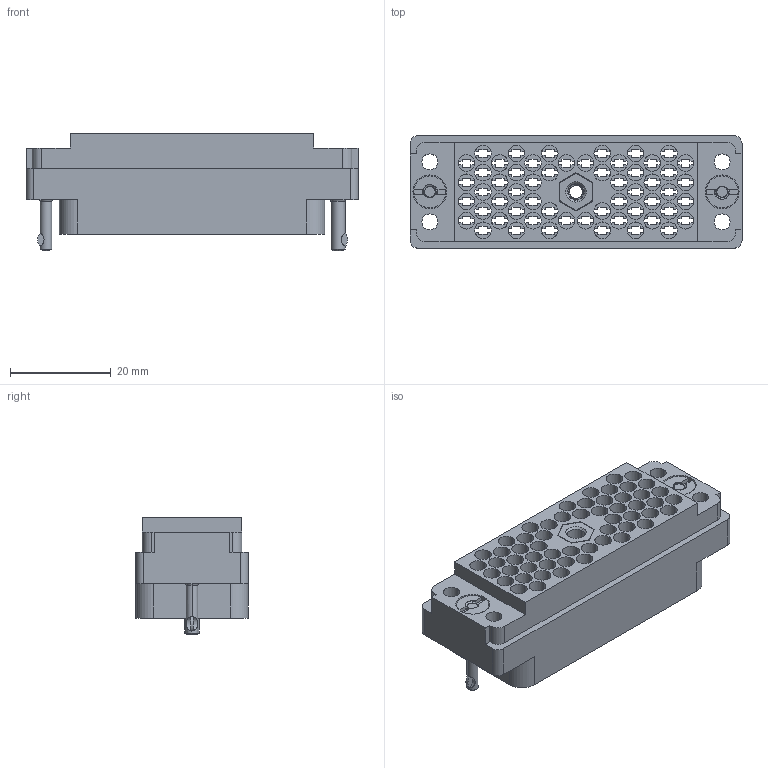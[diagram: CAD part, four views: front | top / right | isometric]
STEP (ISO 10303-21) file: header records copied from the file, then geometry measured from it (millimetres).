
FILE_DESCRIPTION (( 'STEP AP203' ), '1' );
FILE_NAME ('516-056-000-502.STEP', '2020-03-10T04:58:30', ( '' ), ( '' ), 'SwSTEP 2.0', 'SolidWorks 2016', '' );
FILE_SCHEMA (( 'CONFIG_CONTROL_DESIGN' ));
Length unit declared in the file: inch
Products named in the file (6): 516-222-038-102_057; 516-252-035-100_516-252-035-100; 516-252-021-102_056; 516-222-038-102_056; 516 Plug Insulator_056; 516-056-000-502
Assembly tree (6 placements, depth 2):
  516-056-000-502
    516 Plug Insulator_056
    516-252-021-102_056  x2
    516-222-038-102_056
    516-252-035-100_516-252-035-100
    516-222-038-102_057
Bounding box: 65.81 x 22.25 x 23.37 mm (x, y, z)
Volume: 11800.2 mm3; surface area: 16417.7 mm2
Topology: 6 solids, 6 shells, 1455 faces, 4200 edges, 2780 vertices
Faces by surface type: plane 952, cylinder 411, cone 46, bspline 42, torus 4
Entity records: 54195 total; most frequent: CARTESIAN_POINT 15510, ORIENTED_EDGE 8220, DIRECTION 7694, EDGE_CURVE 4110, VECTOR 2876, LINE 2876, VERTEX_POINT 2720, AXIS2_PLACEMENT_3D 2409
